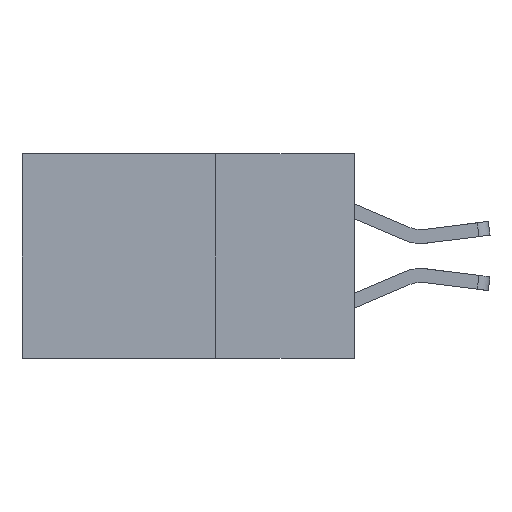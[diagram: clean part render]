
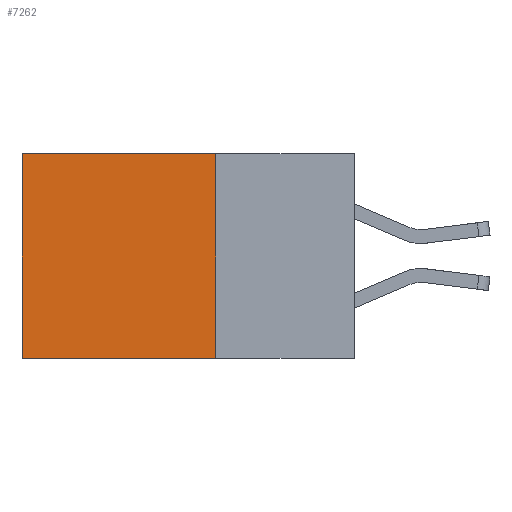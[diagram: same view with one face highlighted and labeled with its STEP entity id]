
A CAD part, left-side view. The second image highlights one B-rep face of the part: STEP entity #7262.
In plain terms, the highlighted planar face has unit normal (-1, 0, 0).
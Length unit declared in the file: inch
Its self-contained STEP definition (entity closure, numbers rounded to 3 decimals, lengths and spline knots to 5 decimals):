
#86 = DIRECTION ( 'NONE',  ( 0., 0., -1. ) ) ;
#331 = FACE_OUTER_BOUND ( 'NONE', #5466, .T. ) ;
#478 = VECTOR ( 'NONE', #1096, 39.37008 ) ;
#531 = VECTOR ( 'NONE', #1424, 39.37008 ) ;
#552 = EDGE_CURVE ( 'NONE', #4916, #6606, #2790, .T. ) ;
#831 = CARTESIAN_POINT ( 'NONE',  ( 0.2615, 0.6, -0.37 ) ) ;
#872 = CARTESIAN_POINT ( 'NONE',  ( 0.2615, 0.25, 0. ) ) ;
#894 = CARTESIAN_POINT ( 'NONE',  ( 0.2615, 0.6, -0.37 ) ) ;
#1081 = DIRECTION ( 'NONE',  ( 0., 0., -1. ) ) ;
#1096 = DIRECTION ( 'NONE',  ( 0., 1., 0. ) ) ;
#1424 = DIRECTION ( 'NONE',  ( 0., 1., 0. ) ) ;
#1474 = LINE ( 'NONE', #1525, #531 ) ;
#1525 = CARTESIAN_POINT ( 'NONE',  ( 0.2615, 0.25, 0. ) ) ;
#1818 = ORIENTED_EDGE ( 'NONE', *, *, #5150, .F. ) ;
#2462 = VERTEX_POINT ( 'NONE', #3869 ) ;
#2478 = VERTEX_POINT ( 'NONE', #872 ) ;
#2625 = ORIENTED_EDGE ( 'NONE', *, *, #4231, .T. ) ;
#2790 = LINE ( 'NONE', #8100, #478 ) ;
#3731 = CARTESIAN_POINT ( 'NONE',  ( 0.2615, 0.25, -0.37 ) ) ;
#3869 = CARTESIAN_POINT ( 'NONE',  ( 0.2615, 0.6, 0. ) ) ;
#4231 = EDGE_CURVE ( 'NONE', #2478, #2462, #1474, .T. ) ;
#4487 = LINE ( 'NONE', #3731, #7375 ) ;
#4587 = DIRECTION ( 'NONE',  ( 0., 0., -1. ) ) ;
#4916 = VERTEX_POINT ( 'NONE', #5741 ) ;
#5026 = ORIENTED_EDGE ( 'NONE', *, *, #7152, .T. ) ;
#5150 = EDGE_CURVE ( 'NONE', #2478, #4916, #4487, .T. ) ;
#5255 = ORIENTED_EDGE ( 'NONE', *, *, #552, .F. ) ;
#5466 = EDGE_LOOP ( 'NONE', ( #5026, #5255, #1818, #2625 ) ) ;
#5741 = CARTESIAN_POINT ( 'NONE',  ( 0.2615, 0.25, -0.37 ) ) ;
#6606 = VERTEX_POINT ( 'NONE', #894 ) ;
#6931 = AXIS2_PLACEMENT_3D ( 'NONE', #8783, #8737, #1081 ) ;
#6976 = LINE ( 'NONE', #831, #9336 ) ;
#7152 = EDGE_CURVE ( 'NONE', #2462, #6606, #6976, .T. ) ;
#7262 = ADVANCED_FACE ( 'NONE', ( #331 ), #7937, .F. ) ;
#7375 = VECTOR ( 'NONE', #4587, 39.37008 ) ;
#7937 = PLANE ( 'NONE',  #6931 ) ;
#8100 = CARTESIAN_POINT ( 'NONE',  ( 0.2615, 0.25, -0.37 ) ) ;
#8737 = DIRECTION ( 'NONE',  ( 1., 0., 0. ) ) ;
#8783 = CARTESIAN_POINT ( 'NONE',  ( 0.2615, 0.25, -0.37 ) ) ;
#9336 = VECTOR ( 'NONE', #86, 39.37008 ) ;
